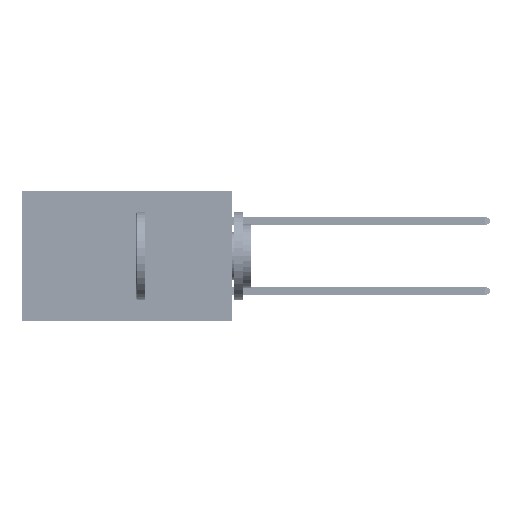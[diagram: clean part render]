
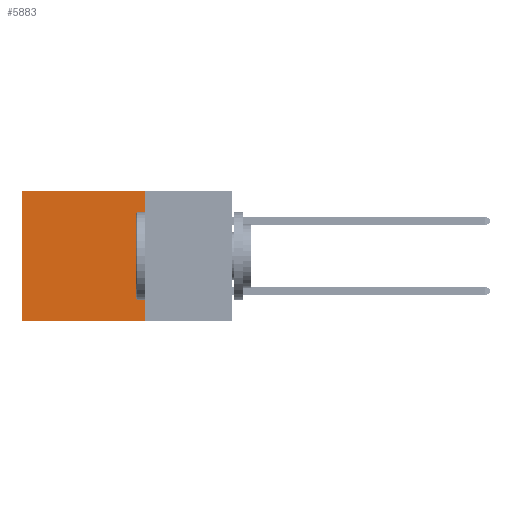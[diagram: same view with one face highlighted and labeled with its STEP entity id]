
A CAD part, left-side view. The second image highlights one B-rep face of the part: STEP entity #5883.
In plain terms, the highlighted planar face has unit normal (-1, 0, 0).
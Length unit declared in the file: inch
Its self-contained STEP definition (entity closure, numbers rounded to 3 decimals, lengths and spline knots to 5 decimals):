
#2440 = PLANE ( 'NONE',  #9837 ) ;
#4687 = VERTEX_POINT ( 'NONE', #16980 ) ;
#5883 = ADVANCED_FACE ( 'NONE', ( #27362 ), #2440, .F. ) ;
#6147 = DIRECTION ( 'NONE',  ( 1., 0., 0. ) ) ;
#8398 = VECTOR ( 'NONE', #31717, 39.37008 ) ;
#9026 = EDGE_CURVE ( 'NONE', #12016, #43745, #39717, .T. ) ;
#9837 = AXIS2_PLACEMENT_3D ( 'NONE', #46144, #6147, #31703 ) ;
#12016 = VERTEX_POINT ( 'NONE', #15419 ) ;
#12642 = DIRECTION ( 'NONE',  ( 0., 1., 0. ) ) ;
#14433 = DIRECTION ( 'NONE',  ( 0., 1., 0. ) ) ;
#15419 = CARTESIAN_POINT ( 'NONE',  ( 0.2875, 0.25, 0. ) ) ;
#16980 = CARTESIAN_POINT ( 'NONE',  ( 0.2875, 0.25, -0.37 ) ) ;
#18090 = CARTESIAN_POINT ( 'NONE',  ( 0.2875, 0.25, -0.37 ) ) ;
#18897 = LINE ( 'NONE', #24021, #46774 ) ;
#19195 = VECTOR ( 'NONE', #12642, 39.37008 ) ;
#21527 = LINE ( 'NONE', #28041, #8398 ) ;
#22193 = VERTEX_POINT ( 'NONE', #36621 ) ;
#23908 = ORIENTED_EDGE ( 'NONE', *, *, #34660, .T. ) ;
#24021 = CARTESIAN_POINT ( 'NONE',  ( 0.2875, 0.25, 0. ) ) ;
#24432 = EDGE_CURVE ( 'NONE', #4687, #22193, #25127, .T. ) ;
#25127 = LINE ( 'NONE', #18090, #43366 ) ;
#25975 = EDGE_CURVE ( 'NONE', #12016, #4687, #18897, .T. ) ;
#26894 = EDGE_LOOP ( 'NONE', ( #23908, #46452, #42119, #29522 ) ) ;
#27362 = FACE_OUTER_BOUND ( 'NONE', #26894, .T. ) ;
#27745 = DIRECTION ( 'NONE',  ( 0., 0., -1. ) ) ;
#28041 = CARTESIAN_POINT ( 'NONE',  ( 0.2875, 0.6, 0. ) ) ;
#28145 = CARTESIAN_POINT ( 'NONE',  ( 0.2875, 0.6, 0. ) ) ;
#29522 = ORIENTED_EDGE ( 'NONE', *, *, #9026, .T. ) ;
#31703 = DIRECTION ( 'NONE',  ( 0., 0., -1. ) ) ;
#31717 = DIRECTION ( 'NONE',  ( 0., 0., -1. ) ) ;
#34660 = EDGE_CURVE ( 'NONE', #43745, #22193, #21527, .T. ) ;
#36621 = CARTESIAN_POINT ( 'NONE',  ( 0.2875, 0.6, -0.37 ) ) ;
#39717 = LINE ( 'NONE', #45250, #19195 ) ;
#42119 = ORIENTED_EDGE ( 'NONE', *, *, #25975, .F. ) ;
#43366 = VECTOR ( 'NONE', #14433, 39.37008 ) ;
#43745 = VERTEX_POINT ( 'NONE', #28145 ) ;
#45250 = CARTESIAN_POINT ( 'NONE',  ( 0.2875, 0.25, 0. ) ) ;
#46144 = CARTESIAN_POINT ( 'NONE',  ( 0.2875, 0.25, 0. ) ) ;
#46452 = ORIENTED_EDGE ( 'NONE', *, *, #24432, .F. ) ;
#46774 = VECTOR ( 'NONE', #27745, 39.37008 ) ;
